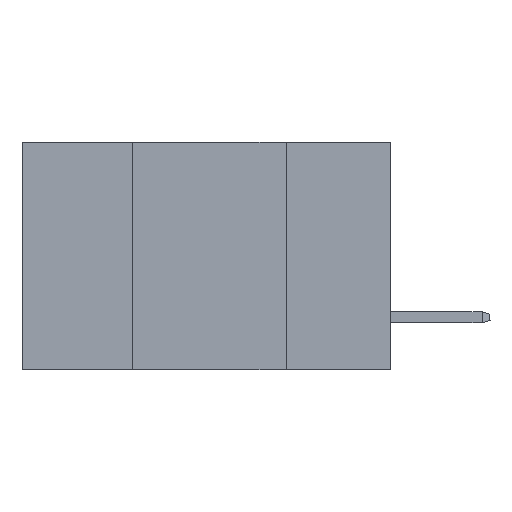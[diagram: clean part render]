
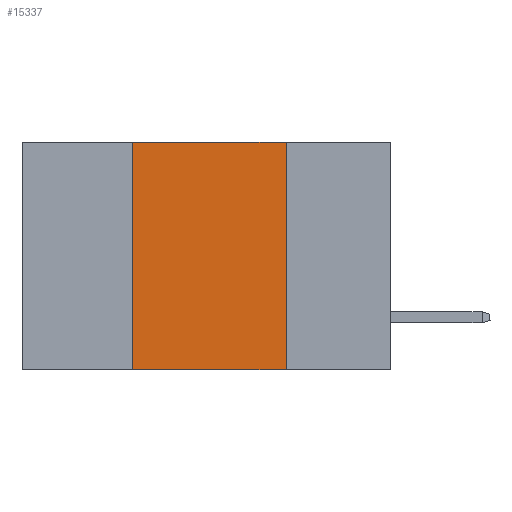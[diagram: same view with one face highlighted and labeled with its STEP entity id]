
A CAD part, left-side view. The second image highlights one B-rep face of the part: STEP entity #15337.
In plain terms, the highlighted planar face has unit normal (-1, 0, 0).
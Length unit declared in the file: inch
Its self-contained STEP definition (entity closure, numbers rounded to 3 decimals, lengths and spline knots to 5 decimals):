
#403 = CARTESIAN_POINT ( 'NONE',  ( 0., 0.6, 0. ) ) ;
#2386 = LINE ( 'NONE', #17016, #8075 ) ;
#3141 = VECTOR ( 'NONE', #13785, 39.37008 ) ;
#5537 = VECTOR ( 'NONE', #35537, 39.37008 ) ;
#6509 = AXIS2_PLACEMENT_3D ( 'NONE', #403, #25755, #11428 ) ;
#6773 = LINE ( 'NONE', #24384, #15102 ) ;
#6901 = VERTEX_POINT ( 'NONE', #34149 ) ;
#7237 = VERTEX_POINT ( 'NONE', #23901 ) ;
#7675 = CARTESIAN_POINT ( 'NONE',  ( 0., 0.17, 0. ) ) ;
#8075 = VECTOR ( 'NONE', #22582, 39.37008 ) ;
#8263 = CARTESIAN_POINT ( 'NONE',  ( 0., 0.6, 0. ) ) ;
#9746 = EDGE_LOOP ( 'NONE', ( #31880, #11399, #34662, #22230 ) ) ;
#10070 = EDGE_CURVE ( 'NONE', #7237, #6901, #2386, .T. ) ;
#10157 = CARTESIAN_POINT ( 'NONE',  ( 0., 0.17, 0. ) ) ;
#10684 = VERTEX_POINT ( 'NONE', #22196 ) ;
#11399 = ORIENTED_EDGE ( 'NONE', *, *, #26675, .F. ) ;
#11428 = DIRECTION ( 'NONE',  ( 0., 0., -1. ) ) ;
#11909 = PLANE ( 'NONE',  #6509 ) ;
#13785 = DIRECTION ( 'NONE',  ( 0., -1., 0. ) ) ;
#15102 = VECTOR ( 'NONE', #23910, 39.37008 ) ;
#15337 = ADVANCED_FACE ( 'NONE', ( #22395 ), #11909, .F. ) ;
#17016 = CARTESIAN_POINT ( 'NONE',  ( 0., 0.42, 0. ) ) ;
#20380 = LINE ( 'NONE', #7675, #5537 ) ;
#21698 = EDGE_CURVE ( 'NONE', #30964, #10684, #20380, .T. ) ;
#22196 = CARTESIAN_POINT ( 'NONE',  ( 0., 0.17, -0.37 ) ) ;
#22230 = ORIENTED_EDGE ( 'NONE', *, *, #24387, .T. ) ;
#22395 = FACE_OUTER_BOUND ( 'NONE', #9746, .T. ) ;
#22582 = DIRECTION ( 'NONE',  ( 0., 0., 1. ) ) ;
#23901 = CARTESIAN_POINT ( 'NONE',  ( 0., 0.42, -0.37 ) ) ;
#23910 = DIRECTION ( 'NONE',  ( 0., -1., 0. ) ) ;
#24384 = CARTESIAN_POINT ( 'NONE',  ( 0., 0.6, -0.37 ) ) ;
#24387 = EDGE_CURVE ( 'NONE', #7237, #10684, #6773, .T. ) ;
#25361 = LINE ( 'NONE', #8263, #3141 ) ;
#25755 = DIRECTION ( 'NONE',  ( 1., 0., 0. ) ) ;
#26675 = EDGE_CURVE ( 'NONE', #6901, #30964, #25361, .T. ) ;
#30964 = VERTEX_POINT ( 'NONE', #10157 ) ;
#31880 = ORIENTED_EDGE ( 'NONE', *, *, #21698, .F. ) ;
#34149 = CARTESIAN_POINT ( 'NONE',  ( 0., 0.42, 0. ) ) ;
#34662 = ORIENTED_EDGE ( 'NONE', *, *, #10070, .F. ) ;
#35537 = DIRECTION ( 'NONE',  ( 0., 0., -1. ) ) ;
